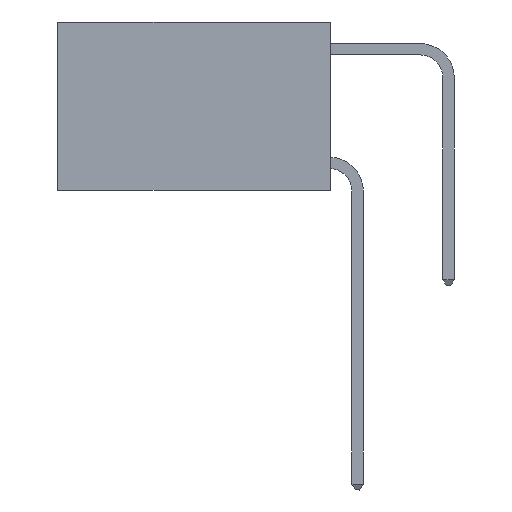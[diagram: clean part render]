
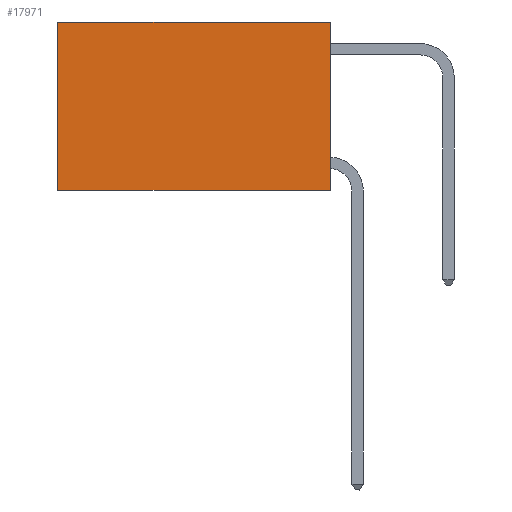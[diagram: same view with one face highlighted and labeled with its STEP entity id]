
A CAD part, left-side view. The second image highlights one B-rep face of the part: STEP entity #17971.
In plain terms, the highlighted planar face has unit normal (-1, 0, 0).
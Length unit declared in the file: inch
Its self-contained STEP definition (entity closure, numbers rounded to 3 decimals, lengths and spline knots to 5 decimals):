
#144 = ORIENTED_EDGE ( 'NONE', *, *, #11295, .F. ) ;
#777 = VECTOR ( 'NONE', #6488, 39.37008 ) ;
#818 = DIRECTION ( 'NONE',  ( 0., 0., -1. ) ) ;
#2006 = DIRECTION ( 'NONE',  ( 0., 0., -1. ) ) ;
#2485 = DIRECTION ( 'NONE',  ( 0., 1., 0. ) ) ;
#2826 = ORIENTED_EDGE ( 'NONE', *, *, #12877, .F. ) ;
#2902 = DIRECTION ( 'NONE',  ( 0., 0., -1. ) ) ;
#3230 = LINE ( 'NONE', #5264, #17988 ) ;
#3552 = EDGE_CURVE ( 'NONE', #5374, #16834, #14529, .T. ) ;
#4184 = CARTESIAN_POINT ( 'NONE',  ( 0.2625, 0.6, 0. ) ) ;
#5264 = CARTESIAN_POINT ( 'NONE',  ( 0.2625, 0., -0.37 ) ) ;
#5374 = VERTEX_POINT ( 'NONE', #4184 ) ;
#6418 = CARTESIAN_POINT ( 'NONE',  ( 0.2625, 0., 0. ) ) ;
#6488 = DIRECTION ( 'NONE',  ( 0., 1., 0. ) ) ;
#7880 = VERTEX_POINT ( 'NONE', #17882 ) ;
#9052 = CARTESIAN_POINT ( 'NONE',  ( 0.2625, 0.6, -0.37 ) ) ;
#9286 = DIRECTION ( 'NONE',  ( 1., 0., 0. ) ) ;
#9331 = VERTEX_POINT ( 'NONE', #17765 ) ;
#9992 = FACE_OUTER_BOUND ( 'NONE', #10541, .T. ) ;
#10417 = CARTESIAN_POINT ( 'NONE',  ( 0.2625, 0., 0. ) ) ;
#10541 = EDGE_LOOP ( 'NONE', ( #14417, #144, #2826, #17053 ) ) ;
#10900 = VECTOR ( 'NONE', #2902, 39.37008 ) ;
#11198 = EDGE_CURVE ( 'NONE', #7880, #5374, #15611, .T. ) ;
#11295 = EDGE_CURVE ( 'NONE', #9331, #16834, #3230, .T. ) ;
#11435 = VECTOR ( 'NONE', #2006, 39.37008 ) ;
#11988 = PLANE ( 'NONE',  #17506 ) ;
#12877 = EDGE_CURVE ( 'NONE', #7880, #9331, #17262, .T. ) ;
#14417 = ORIENTED_EDGE ( 'NONE', *, *, #3552, .T. ) ;
#14529 = LINE ( 'NONE', #14924, #10900 ) ;
#14924 = CARTESIAN_POINT ( 'NONE',  ( 0.2625, 0.6, 0. ) ) ;
#15611 = LINE ( 'NONE', #6418, #777 ) ;
#16834 = VERTEX_POINT ( 'NONE', #9052 ) ;
#17053 = ORIENTED_EDGE ( 'NONE', *, *, #11198, .T. ) ;
#17262 = LINE ( 'NONE', #10417, #11435 ) ;
#17495 = CARTESIAN_POINT ( 'NONE',  ( 0.2625, 0., 0. ) ) ;
#17506 = AXIS2_PLACEMENT_3D ( 'NONE', #17495, #9286, #818 ) ;
#17765 = CARTESIAN_POINT ( 'NONE',  ( 0.2625, 0., -0.37 ) ) ;
#17882 = CARTESIAN_POINT ( 'NONE',  ( 0.2625, 0., 0. ) ) ;
#17971 = ADVANCED_FACE ( 'NONE', ( #9992 ), #11988, .F. ) ;
#17988 = VECTOR ( 'NONE', #2485, 39.37008 ) ;
